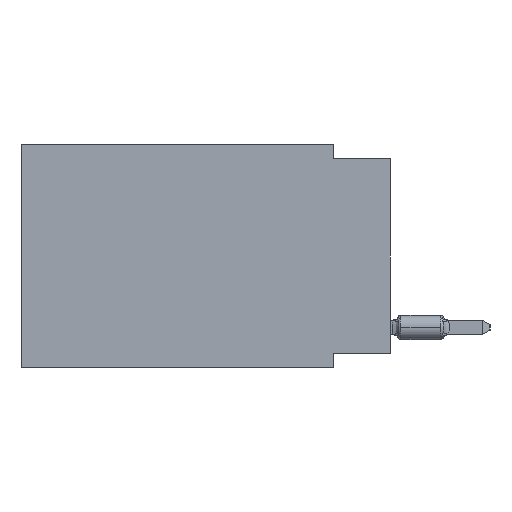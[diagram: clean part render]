
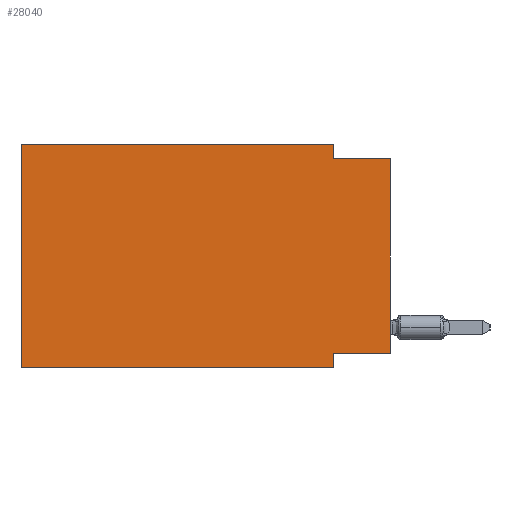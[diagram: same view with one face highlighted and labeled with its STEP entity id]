
A CAD part, left-side view. The second image highlights one B-rep face of the part: STEP entity #28040.
In plain terms, the highlighted planar face has unit normal (-1, 0, 0).
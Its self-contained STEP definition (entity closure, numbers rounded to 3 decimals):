
#2085 = VERTEX_POINT ( 'NONE', #19407 ) ;
#2535 = DIRECTION ( 'NONE',  ( 0., 0., -1. ) ) ;
#3181 = LINE ( 'NONE', #51000, #4993 ) ;
#3481 = DIRECTION ( 'NONE',  ( 0., 0., -1. ) ) ;
#4993 = VECTOR ( 'NONE', #20078, 1000. ) ;
#5037 = VECTOR ( 'NONE', #36273, 1000. ) ;
#9141 = VECTOR ( 'NONE', #52799, 1000. ) ;
#9842 = LINE ( 'NONE', #35319, #9141 ) ;
#10557 = ORIENTED_EDGE ( 'NONE', *, *, #29377, .F. ) ;
#11822 = VECTOR ( 'NONE', #53513, 1000. ) ;
#13881 = DIRECTION ( 'NONE',  ( 0., -1., 0. ) ) ;
#13895 = CARTESIAN_POINT ( 'NONE',  ( 0., 2.54, 0. ) ) ;
#14201 = ORIENTED_EDGE ( 'NONE', *, *, #51017, .T. ) ;
#14271 = VERTEX_POINT ( 'NONE', #26976 ) ;
#14967 = VERTEX_POINT ( 'NONE', #51995 ) ;
#15426 = LINE ( 'NONE', #38031, #20476 ) ;
#16929 = PLANE ( 'NONE',  #17178 ) ;
#17178 = AXIS2_PLACEMENT_3D ( 'NONE', #56141, #42682, #3481 ) ;
#19106 = CARTESIAN_POINT ( 'NONE',  ( 0., 16.383, 0. ) ) ;
#19407 = CARTESIAN_POINT ( 'NONE',  ( 0., 2.54, -9.271 ) ) ;
#19894 = VERTEX_POINT ( 'NONE', #13895 ) ;
#20042 = ORIENTED_EDGE ( 'NONE', *, *, #51938, .F. ) ;
#20078 = DIRECTION ( 'NONE',  ( 0., -1., 0. ) ) ;
#20476 = VECTOR ( 'NONE', #2535, 1000. ) ;
#20790 = CARTESIAN_POINT ( 'NONE',  ( 0., 2.54, 0. ) ) ;
#21318 = CARTESIAN_POINT ( 'NONE',  ( 0., 16.383, 0. ) ) ;
#22445 = VERTEX_POINT ( 'NONE', #33942 ) ;
#25835 = EDGE_LOOP ( 'NONE', ( #38644, #10557, #20042, #46975, #42429, #14201, #47568, #50684 ) ) ;
#25937 = DIRECTION ( 'NONE',  ( 0., 0., -1. ) ) ;
#26976 = CARTESIAN_POINT ( 'NONE',  ( 0., 2.54, -0.635 ) ) ;
#27468 = CARTESIAN_POINT ( 'NONE',  ( 0., 0., -9.271 ) ) ;
#28040 = ADVANCED_FACE ( 'NONE', ( #42399 ), #16929, .F. ) ;
#29377 = EDGE_CURVE ( 'NONE', #14271, #53413, #35611, .T. ) ;
#30371 = EDGE_CURVE ( 'NONE', #14967, #2085, #36040, .T. ) ;
#33942 = CARTESIAN_POINT ( 'NONE',  ( 0., 16.383, 0. ) ) ;
#34275 = VECTOR ( 'NONE', #25937, 1000. ) ;
#34483 = VERTEX_POINT ( 'NONE', #49076 ) ;
#35029 = LINE ( 'NONE', #21318, #47224 ) ;
#35190 = CARTESIAN_POINT ( 'NONE',  ( 0., 2.54, -9.906 ) ) ;
#35319 = CARTESIAN_POINT ( 'NONE',  ( 0., 0., 0. ) ) ;
#35611 = LINE ( 'NONE', #53095, #48325 ) ;
#36040 = LINE ( 'NONE', #27468, #11822 ) ;
#36273 = DIRECTION ( 'NONE',  ( 0., -1., 0. ) ) ;
#38031 = CARTESIAN_POINT ( 'NONE',  ( 0., 2.54, -9.906 ) ) ;
#38644 = ORIENTED_EDGE ( 'NONE', *, *, #56383, .T. ) ;
#40846 = LINE ( 'NONE', #19106, #5037 ) ;
#42399 = FACE_OUTER_BOUND ( 'NONE', #25835, .T. ) ;
#42429 = ORIENTED_EDGE ( 'NONE', *, *, #46421, .F. ) ;
#42682 = DIRECTION ( 'NONE',  ( 1., 0., 0. ) ) ;
#43119 = LINE ( 'NONE', #20790, #34275 ) ;
#46421 = EDGE_CURVE ( 'NONE', #34483, #22445, #35029, .T. ) ;
#46801 = CARTESIAN_POINT ( 'NONE',  ( 0., 0., -0.635 ) ) ;
#46975 = ORIENTED_EDGE ( 'NONE', *, *, #51639, .F. ) ;
#47224 = VECTOR ( 'NONE', #54904, 1000. ) ;
#47568 = ORIENTED_EDGE ( 'NONE', *, *, #50140, .F. ) ;
#48325 = VECTOR ( 'NONE', #13881, 1000. ) ;
#48788 = VERTEX_POINT ( 'NONE', #35190 ) ;
#49076 = CARTESIAN_POINT ( 'NONE',  ( 0., 16.383, -9.906 ) ) ;
#50140 = EDGE_CURVE ( 'NONE', #2085, #48788, #15426, .T. ) ;
#50684 = ORIENTED_EDGE ( 'NONE', *, *, #30371, .F. ) ;
#51000 = CARTESIAN_POINT ( 'NONE',  ( 0., 16.383, -9.906 ) ) ;
#51017 = EDGE_CURVE ( 'NONE', #34483, #48788, #3181, .T. ) ;
#51639 = EDGE_CURVE ( 'NONE', #22445, #19894, #40846, .T. ) ;
#51938 = EDGE_CURVE ( 'NONE', #19894, #14271, #43119, .T. ) ;
#51995 = CARTESIAN_POINT ( 'NONE',  ( 0., 0., -9.271 ) ) ;
#52799 = DIRECTION ( 'NONE',  ( 0., 0., 1. ) ) ;
#53095 = CARTESIAN_POINT ( 'NONE',  ( 0., 0., -0.635 ) ) ;
#53413 = VERTEX_POINT ( 'NONE', #46801 ) ;
#53513 = DIRECTION ( 'NONE',  ( 0., 1., 0. ) ) ;
#54904 = DIRECTION ( 'NONE',  ( 0., 0., 1. ) ) ;
#56141 = CARTESIAN_POINT ( 'NONE',  ( 0., 16.383, 0. ) ) ;
#56383 = EDGE_CURVE ( 'NONE', #14967, #53413, #9842, .T. ) ;
